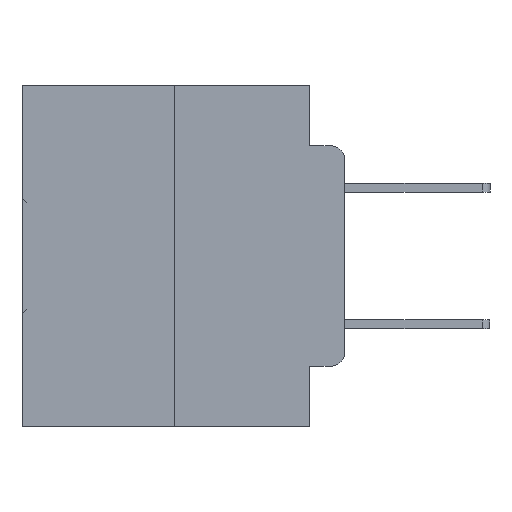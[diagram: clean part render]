
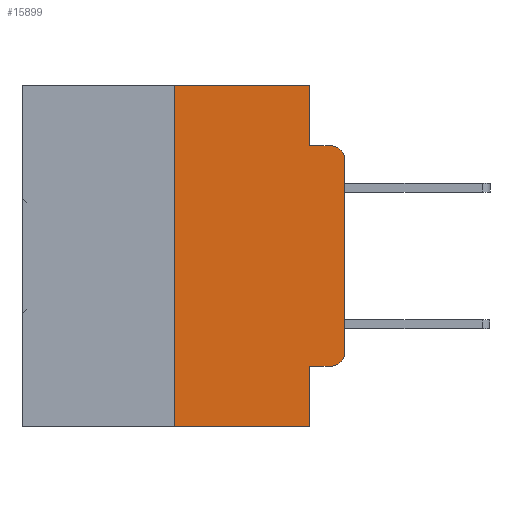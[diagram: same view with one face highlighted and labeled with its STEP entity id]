
A CAD part, left-side view. The second image highlights one B-rep face of the part: STEP entity #15899.
In plain terms, the highlighted planar face has unit normal (-1, 0, 0).
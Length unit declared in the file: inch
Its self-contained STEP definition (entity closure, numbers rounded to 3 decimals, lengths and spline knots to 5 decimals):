
#51 = CARTESIAN_POINT ( 'NONE',  ( 0., 0.473, 0. ) ) ;
#131 = CARTESIAN_POINT ( 'NONE',  ( 0., 0.473, -0.5 ) ) ;
#165 = CARTESIAN_POINT ( 'NONE',  ( 0., 0.02, -0.0885 ) ) ;
#303 = EDGE_CURVE ( 'NONE', #7929, #26067, #16884, .T. ) ;
#486 = CARTESIAN_POINT ( 'NONE',  ( 0., 0.051, -0.0885 ) ) ;
#981 = ORIENTED_EDGE ( 'NONE', *, *, #30224, .F. ) ;
#1279 = VECTOR ( 'NONE', #27740, 39.37008 ) ;
#1913 = CARTESIAN_POINT ( 'NONE',  ( 0., 0.051, 0. ) ) ;
#2199 = AXIS2_PLACEMENT_3D ( 'NONE', #51, #18519, #2754 ) ;
#2754 = DIRECTION ( 'NONE',  ( 0., 0., -1. ) ) ;
#3195 = DIRECTION ( 'NONE',  ( -1., 0., 0. ) ) ;
#3232 = ORIENTED_EDGE ( 'NONE', *, *, #16578, .T. ) ;
#3480 = DIRECTION ( 'NONE',  ( 0., 0., -1. ) ) ;
#3614 = CARTESIAN_POINT ( 'NONE',  ( 0., 0.051, -0.5 ) ) ;
#4218 = CARTESIAN_POINT ( 'NONE',  ( 0., 0.473, 0. ) ) ;
#4326 = EDGE_CURVE ( 'NONE', #23134, #26067, #29600, .T. ) ;
#4766 = CARTESIAN_POINT ( 'NONE',  ( 0., 0.051, 0. ) ) ;
#5074 = CARTESIAN_POINT ( 'NONE',  ( 0., 0.25, 0. ) ) ;
#5093 = DIRECTION ( 'NONE',  ( 0., 0., 1. ) ) ;
#5218 = DIRECTION ( 'NONE',  ( 0., 0., 1. ) ) ;
#5330 = LINE ( 'NONE', #486, #11550 ) ;
#5611 = ORIENTED_EDGE ( 'NONE', *, *, #25603, .F. ) ;
#5773 = EDGE_CURVE ( 'NONE', #7929, #6666, #19002, .T. ) ;
#6356 = ORIENTED_EDGE ( 'NONE', *, *, #4326, .T. ) ;
#6666 = VERTEX_POINT ( 'NONE', #26126 ) ;
#7389 = DIRECTION ( 'NONE',  ( -1., 0., 0. ) ) ;
#7848 = VECTOR ( 'NONE', #12668, 39.37008 ) ;
#7867 = VERTEX_POINT ( 'NONE', #26284 ) ;
#7929 = VERTEX_POINT ( 'NONE', #29229 ) ;
#8704 = LINE ( 'NONE', #4766, #7848 ) ;
#9908 = VECTOR ( 'NONE', #3480, 39.37008 ) ;
#10495 = LINE ( 'NONE', #13194, #12979 ) ;
#10656 = ORIENTED_EDGE ( 'NONE', *, *, #21345, .F. ) ;
#10924 = VERTEX_POINT ( 'NONE', #5074 ) ;
#11034 = VERTEX_POINT ( 'NONE', #165 ) ;
#11241 = VECTOR ( 'NONE', #31679, 39.37008 ) ;
#11550 = VECTOR ( 'NONE', #31903, 39.37008 ) ;
#12668 = DIRECTION ( 'NONE',  ( 0., 0., -1. ) ) ;
#12968 = CARTESIAN_POINT ( 'NONE',  ( 0., 0.25, 0. ) ) ;
#12979 = VECTOR ( 'NONE', #5218, 39.37008 ) ;
#13194 = CARTESIAN_POINT ( 'NONE',  ( 0., 0., 0. ) ) ;
#14096 = ORIENTED_EDGE ( 'NONE', *, *, #5773, .T. ) ;
#15346 = VERTEX_POINT ( 'NONE', #29173 ) ;
#15849 = CARTESIAN_POINT ( 'NONE',  ( 0., 0.25, -0.5 ) ) ;
#15899 = ADVANCED_FACE ( 'NONE', ( #28236 ), #26190, .F. ) ;
#16578 = EDGE_CURVE ( 'NONE', #15346, #11034, #30232, .T. ) ;
#16650 = ORIENTED_EDGE ( 'NONE', *, *, #303, .F. ) ;
#16884 = LINE ( 'NONE', #1913, #9908 ) ;
#18519 = DIRECTION ( 'NONE',  ( 1., 0., 0. ) ) ;
#18936 = CARTESIAN_POINT ( 'NONE',  ( 0., 0.02, -0.1085 ) ) ;
#19002 = LINE ( 'NONE', #25071, #11241 ) ;
#19812 = ORIENTED_EDGE ( 'NONE', *, *, #29531, .F. ) ;
#19882 = EDGE_LOOP ( 'NONE', ( #24026, #3232, #10656, #19812, #5611, #981, #6356, #16650, #14096, #21401 ) ) ;
#20512 = VECTOR ( 'NONE', #5093, 39.37008 ) ;
#21006 = DIRECTION ( 'NONE',  ( 0., -1., 0. ) ) ;
#21345 = EDGE_CURVE ( 'NONE', #7867, #11034, #5330, .T. ) ;
#21401 = ORIENTED_EDGE ( 'NONE', *, *, #27309, .T. ) ;
#21569 = DIRECTION ( 'NONE',  ( 0., 0., -1. ) ) ;
#22490 = AXIS2_PLACEMENT_3D ( 'NONE', #23066, #7389, #25623 ) ;
#23066 = CARTESIAN_POINT ( 'NONE',  ( 0., 0.02, -0.3915 ) ) ;
#23134 = VERTEX_POINT ( 'NONE', #15849 ) ;
#23502 = VERTEX_POINT ( 'NONE', #24130 ) ;
#23816 = LINE ( 'NONE', #4218, #1279 ) ;
#24026 = ORIENTED_EDGE ( 'NONE', *, *, #33795, .T. ) ;
#24130 = CARTESIAN_POINT ( 'NONE',  ( 0., 0., -0.3915 ) ) ;
#24366 = AXIS2_PLACEMENT_3D ( 'NONE', #18936, #3195, #21569 ) ;
#24491 = CIRCLE ( 'NONE', #22490, 0.02 ) ;
#25071 = CARTESIAN_POINT ( 'NONE',  ( 0., 0.051, -0.4115 ) ) ;
#25603 = EDGE_CURVE ( 'NONE', #10924, #33144, #23816, .T. ) ;
#25623 = DIRECTION ( 'NONE',  ( 0., 0., -1. ) ) ;
#26067 = VERTEX_POINT ( 'NONE', #3614 ) ;
#26126 = CARTESIAN_POINT ( 'NONE',  ( 0., 0.02, -0.4115 ) ) ;
#26190 = PLANE ( 'NONE',  #2199 ) ;
#26284 = CARTESIAN_POINT ( 'NONE',  ( 0., 0.051, -0.0885 ) ) ;
#27309 = EDGE_CURVE ( 'NONE', #6666, #23502, #24491, .T. ) ;
#27368 = LINE ( 'NONE', #12968, #20512 ) ;
#27740 = DIRECTION ( 'NONE',  ( 0., -1., 0. ) ) ;
#28236 = FACE_OUTER_BOUND ( 'NONE', #19882, .T. ) ;
#29173 = CARTESIAN_POINT ( 'NONE',  ( 0., 0., -0.1085 ) ) ;
#29229 = CARTESIAN_POINT ( 'NONE',  ( 0., 0.051, -0.4115 ) ) ;
#29531 = EDGE_CURVE ( 'NONE', #33144, #7867, #8704, .T. ) ;
#29600 = LINE ( 'NONE', #131, #30407 ) ;
#30224 = EDGE_CURVE ( 'NONE', #23134, #10924, #27368, .T. ) ;
#30232 = CIRCLE ( 'NONE', #24366, 0.02 ) ;
#30407 = VECTOR ( 'NONE', #21006, 39.37008 ) ;
#30440 = CARTESIAN_POINT ( 'NONE',  ( 0., 0.051, 0. ) ) ;
#31679 = DIRECTION ( 'NONE',  ( 0., -1., 0. ) ) ;
#31903 = DIRECTION ( 'NONE',  ( 0., -1., 0. ) ) ;
#33144 = VERTEX_POINT ( 'NONE', #30440 ) ;
#33795 = EDGE_CURVE ( 'NONE', #23502, #15346, #10495, .T. ) ;
